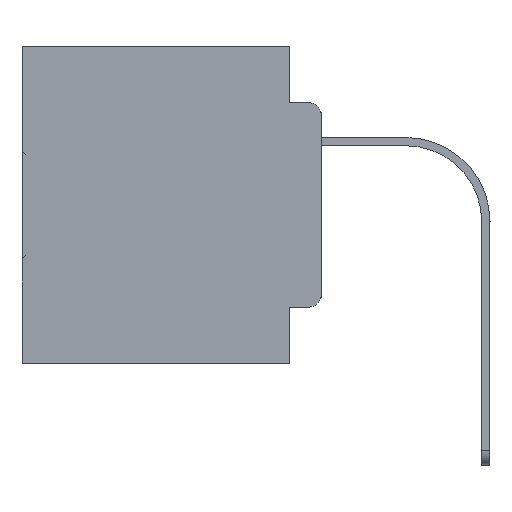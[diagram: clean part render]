
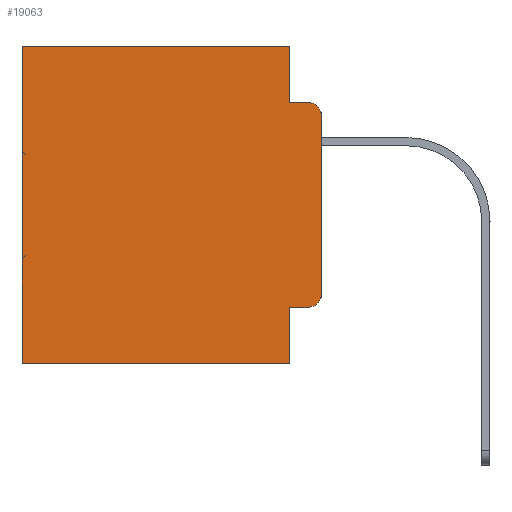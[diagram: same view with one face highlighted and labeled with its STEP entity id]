
A CAD part, left-side view. The second image highlights one B-rep face of the part: STEP entity #19063.
In plain terms, the highlighted planar face has unit normal (-1, 0, 0).
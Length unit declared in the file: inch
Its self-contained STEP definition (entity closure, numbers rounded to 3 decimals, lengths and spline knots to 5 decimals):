
#808 = ORIENTED_EDGE ( 'NONE', *, *, #6515, .T. ) ;
#1095 = DIRECTION ( 'NONE',  ( 0., 1., 0. ) ) ;
#1232 = VERTEX_POINT ( 'NONE', #30525 ) ;
#2354 = CARTESIAN_POINT ( 'NONE',  ( 0.298, 0.051, -0.0885 ) ) ;
#2371 = CARTESIAN_POINT ( 'NONE',  ( 0.298, 0.051, 0. ) ) ;
#2412 = DIRECTION ( 'NONE',  ( 0., -1., 0. ) ) ;
#3174 = ORIENTED_EDGE ( 'NONE', *, *, #6238, .T. ) ;
#3184 = ORIENTED_EDGE ( 'NONE', *, *, #15760, .T. ) ;
#4025 = DIRECTION ( 'NONE',  ( 0., 0., -1. ) ) ;
#4127 = EDGE_CURVE ( 'NONE', #11893, #12818, #22690, .T. ) ;
#4172 = CARTESIAN_POINT ( 'NONE',  ( 0.298, 0., 0. ) ) ;
#5517 = DIRECTION ( 'NONE',  ( 0., 0., -1. ) ) ;
#5539 = VERTEX_POINT ( 'NONE', #5760 ) ;
#5672 = DIRECTION ( 'NONE',  ( 0., 1., 0. ) ) ;
#5677 = CARTESIAN_POINT ( 'NONE',  ( 0.298, 0.051, 0. ) ) ;
#5760 = CARTESIAN_POINT ( 'NONE',  ( 0.298, 0.02, -0.4115 ) ) ;
#5824 = EDGE_CURVE ( 'NONE', #1232, #32477, #28992, .T. ) ;
#6238 = EDGE_CURVE ( 'NONE', #15819, #5539, #28132, .T. ) ;
#6515 = EDGE_CURVE ( 'NONE', #17068, #12818, #33413, .T. ) ;
#6542 = LINE ( 'NONE', #4172, #16859 ) ;
#6808 = EDGE_CURVE ( 'NONE', #5539, #20575, #12797, .T. ) ;
#7074 = LINE ( 'NONE', #32621, #20166 ) ;
#7646 = EDGE_CURVE ( 'NONE', #16778, #11893, #28997, .T. ) ;
#8943 = ORIENTED_EDGE ( 'NONE', *, *, #4127, .F. ) ;
#9308 = CARTESIAN_POINT ( 'NONE',  ( 0.298, 0., 0. ) ) ;
#9816 = ORIENTED_EDGE ( 'NONE', *, *, #6808, .T. ) ;
#10950 = DIRECTION ( 'NONE',  ( 1., 0., 0. ) ) ;
#11893 = VERTEX_POINT ( 'NONE', #2354 ) ;
#12254 = VECTOR ( 'NONE', #2412, 39.37008 ) ;
#12797 = CIRCLE ( 'NONE', #30731, 0.02 ) ;
#12818 = VERTEX_POINT ( 'NONE', #22763 ) ;
#13445 = CARTESIAN_POINT ( 'NONE',  ( 0.298, 0.02, -0.3915 ) ) ;
#13875 = AXIS2_PLACEMENT_3D ( 'NONE', #26416, #10950, #29316 ) ;
#13881 = VECTOR ( 'NONE', #33134, 39.37008 ) ;
#14012 = PLANE ( 'NONE',  #13875 ) ;
#14683 = DIRECTION ( 'NONE',  ( 0., 0., -1. ) ) ;
#15385 = VECTOR ( 'NONE', #4025, 39.37008 ) ;
#15760 = EDGE_CURVE ( 'NONE', #20785, #32477, #7074, .T. ) ;
#15819 = VERTEX_POINT ( 'NONE', #32269 ) ;
#16090 = ORIENTED_EDGE ( 'NONE', *, *, #7646, .F. ) ;
#16619 = CARTESIAN_POINT ( 'NONE',  ( 0.298, 0.473, 0. ) ) ;
#16778 = VERTEX_POINT ( 'NONE', #2371 ) ;
#16859 = VECTOR ( 'NONE', #1095, 39.37008 ) ;
#17052 = EDGE_CURVE ( 'NONE', #17068, #20575, #27681, .T. ) ;
#17068 = VERTEX_POINT ( 'NONE', #25288 ) ;
#18787 = VECTOR ( 'NONE', #5517, 39.37008 ) ;
#19063 = ADVANCED_FACE ( 'NONE', ( #27091 ), #14012, .F. ) ;
#19644 = CARTESIAN_POINT ( 'NONE',  ( 0.298, 0., -0.3915 ) ) ;
#20166 = VECTOR ( 'NONE', #27330, 39.37008 ) ;
#20464 = DIRECTION ( 'NONE',  ( 0., -1., 0. ) ) ;
#20575 = VERTEX_POINT ( 'NONE', #19644 ) ;
#20785 = VERTEX_POINT ( 'NONE', #16619 ) ;
#21078 = DIRECTION ( 'NONE',  ( 0., 0., -1. ) ) ;
#21182 = VECTOR ( 'NONE', #20464, 39.37008 ) ;
#22319 = CARTESIAN_POINT ( 'NONE',  ( 0.298, 0.02, -0.1085 ) ) ;
#22690 = LINE ( 'NONE', #32744, #21182 ) ;
#22763 = CARTESIAN_POINT ( 'NONE',  ( 0.298, 0.02, -0.0885 ) ) ;
#22812 = DIRECTION ( 'NONE',  ( -1., 0., 0. ) ) ;
#23042 = VECTOR ( 'NONE', #5672, 39.37008 ) ;
#23690 = CARTESIAN_POINT ( 'NONE',  ( 0.298, 0.051, -0.4115 ) ) ;
#23728 = CARTESIAN_POINT ( 'NONE',  ( 0.298, 0., -0.5 ) ) ;
#24125 = EDGE_CURVE ( 'NONE', #16778, #20785, #6542, .T. ) ;
#25288 = CARTESIAN_POINT ( 'NONE',  ( 0.298, 0., -0.1085 ) ) ;
#26416 = CARTESIAN_POINT ( 'NONE',  ( 0.298, 0., 0. ) ) ;
#27091 = FACE_OUTER_BOUND ( 'NONE', #31271, .T. ) ;
#27330 = DIRECTION ( 'NONE',  ( 0., 0., -1. ) ) ;
#27364 = ORIENTED_EDGE ( 'NONE', *, *, #24125, .T. ) ;
#27681 = LINE ( 'NONE', #9308, #15385 ) ;
#27712 = CARTESIAN_POINT ( 'NONE',  ( 0.298, 0.051, 0. ) ) ;
#28132 = LINE ( 'NONE', #23690, #12254 ) ;
#28534 = ORIENTED_EDGE ( 'NONE', *, *, #17052, .F. ) ;
#28913 = DIRECTION ( 'NONE',  ( -1., 0., 0. ) ) ;
#28992 = LINE ( 'NONE', #23728, #23042 ) ;
#28997 = LINE ( 'NONE', #5677, #18787 ) ;
#29316 = DIRECTION ( 'NONE',  ( 0., 0., -1. ) ) ;
#29648 = AXIS2_PLACEMENT_3D ( 'NONE', #22319, #22812, #14683 ) ;
#30525 = CARTESIAN_POINT ( 'NONE',  ( 0.298, 0.051, -0.5 ) ) ;
#30579 = LINE ( 'NONE', #27712, #13881 ) ;
#30731 = AXIS2_PLACEMENT_3D ( 'NONE', #13445, #28913, #21078 ) ;
#30956 = ORIENTED_EDGE ( 'NONE', *, *, #31687, .F. ) ;
#31271 = EDGE_LOOP ( 'NONE', ( #28534, #808, #8943, #16090, #27364, #3184, #32814, #30956, #3174, #9816 ) ) ;
#31484 = CARTESIAN_POINT ( 'NONE',  ( 0.298, 0.473, -0.5 ) ) ;
#31687 = EDGE_CURVE ( 'NONE', #15819, #1232, #30579, .T. ) ;
#32269 = CARTESIAN_POINT ( 'NONE',  ( 0.298, 0.051, -0.4115 ) ) ;
#32477 = VERTEX_POINT ( 'NONE', #31484 ) ;
#32621 = CARTESIAN_POINT ( 'NONE',  ( 0.298, 0.473, 0. ) ) ;
#32744 = CARTESIAN_POINT ( 'NONE',  ( 0.298, 0.051, -0.0885 ) ) ;
#32814 = ORIENTED_EDGE ( 'NONE', *, *, #5824, .F. ) ;
#33134 = DIRECTION ( 'NONE',  ( 0., 0., -1. ) ) ;
#33413 = CIRCLE ( 'NONE', #29648, 0.02 ) ;
